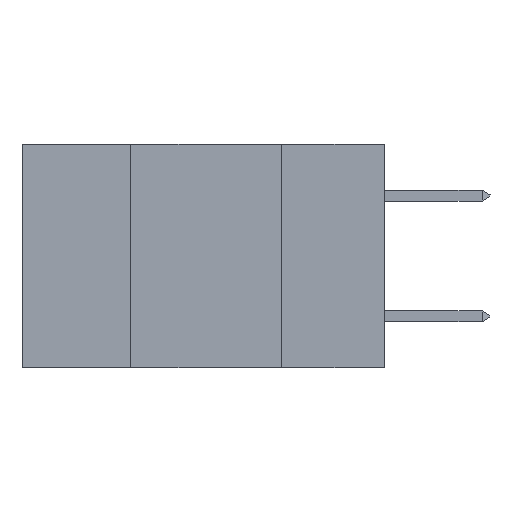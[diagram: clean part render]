
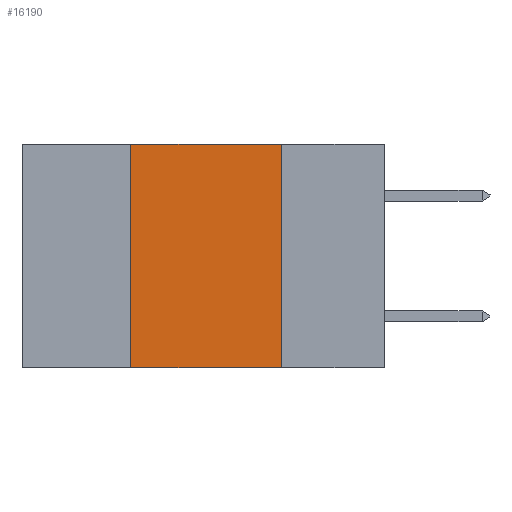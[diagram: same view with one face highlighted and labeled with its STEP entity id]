
A CAD part, left-side view. The second image highlights one B-rep face of the part: STEP entity #16190.
In plain terms, the highlighted planar face has unit normal (-1, 0, 0).
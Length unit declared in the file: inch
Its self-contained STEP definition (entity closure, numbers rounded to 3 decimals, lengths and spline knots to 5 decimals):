
#1674 = VERTEX_POINT ( 'NONE', #35108 ) ;
#2619 = EDGE_CURVE ( 'NONE', #1674, #38603, #7023, .T. ) ;
#5590 = DIRECTION ( 'NONE',  ( 1., 0., 0. ) ) ;
#6896 = EDGE_LOOP ( 'NONE', ( #17165, #7286, #32801, #36832 ) ) ;
#7023 = LINE ( 'NONE', #34423, #29239 ) ;
#7286 = ORIENTED_EDGE ( 'NONE', *, *, #2619, .F. ) ;
#8014 = CARTESIAN_POINT ( 'NONE',  ( 0., 0.17, 0. ) ) ;
#8075 = DIRECTION ( 'NONE',  ( 0., 0., 1. ) ) ;
#10443 = AXIS2_PLACEMENT_3D ( 'NONE', #21588, #5590, #24211 ) ;
#11228 = LINE ( 'NONE', #29429, #27819 ) ;
#12354 = CARTESIAN_POINT ( 'NONE',  ( 0., 0.42, -0.37 ) ) ;
#15298 = VECTOR ( 'NONE', #8075, 39.37008 ) ;
#15427 = DIRECTION ( 'NONE',  ( 0., 0., -1. ) ) ;
#16190 = ADVANCED_FACE ( 'NONE', ( #33397 ), #18201, .F. ) ;
#17165 = ORIENTED_EDGE ( 'NONE', *, *, #18786, .F. ) ;
#18201 = PLANE ( 'NONE',  #10443 ) ;
#18607 = EDGE_CURVE ( 'NONE', #33534, #33284, #11228, .T. ) ;
#18786 = EDGE_CURVE ( 'NONE', #38603, #33284, #26840, .T. ) ;
#21588 = CARTESIAN_POINT ( 'NONE',  ( 0., 0.6, 0. ) ) ;
#23485 = LINE ( 'NONE', #32475, #15298 ) ;
#24211 = DIRECTION ( 'NONE',  ( 0., 0., -1. ) ) ;
#24276 = EDGE_CURVE ( 'NONE', #33534, #1674, #23485, .T. ) ;
#25235 = DIRECTION ( 'NONE',  ( 0., -1., 0. ) ) ;
#26840 = LINE ( 'NONE', #36604, #28453 ) ;
#27819 = VECTOR ( 'NONE', #32622, 39.37008 ) ;
#28453 = VECTOR ( 'NONE', #15427, 39.37008 ) ;
#29239 = VECTOR ( 'NONE', #25235, 39.37008 ) ;
#29429 = CARTESIAN_POINT ( 'NONE',  ( 0., 0.6, -0.37 ) ) ;
#32475 = CARTESIAN_POINT ( 'NONE',  ( 0., 0.42, 0. ) ) ;
#32622 = DIRECTION ( 'NONE',  ( 0., -1., 0. ) ) ;
#32801 = ORIENTED_EDGE ( 'NONE', *, *, #24276, .F. ) ;
#33284 = VERTEX_POINT ( 'NONE', #36811 ) ;
#33397 = FACE_OUTER_BOUND ( 'NONE', #6896, .T. ) ;
#33534 = VERTEX_POINT ( 'NONE', #12354 ) ;
#34423 = CARTESIAN_POINT ( 'NONE',  ( 0., 0.6, 0. ) ) ;
#35108 = CARTESIAN_POINT ( 'NONE',  ( 0., 0.42, 0. ) ) ;
#36604 = CARTESIAN_POINT ( 'NONE',  ( 0., 0.17, 0. ) ) ;
#36811 = CARTESIAN_POINT ( 'NONE',  ( 0., 0.17, -0.37 ) ) ;
#36832 = ORIENTED_EDGE ( 'NONE', *, *, #18607, .T. ) ;
#38603 = VERTEX_POINT ( 'NONE', #8014 ) ;
